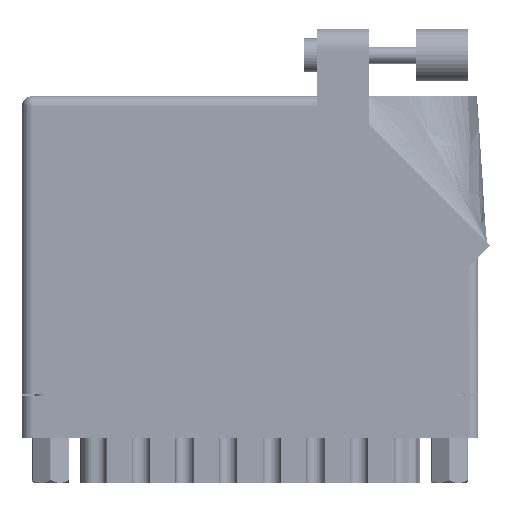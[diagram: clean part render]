
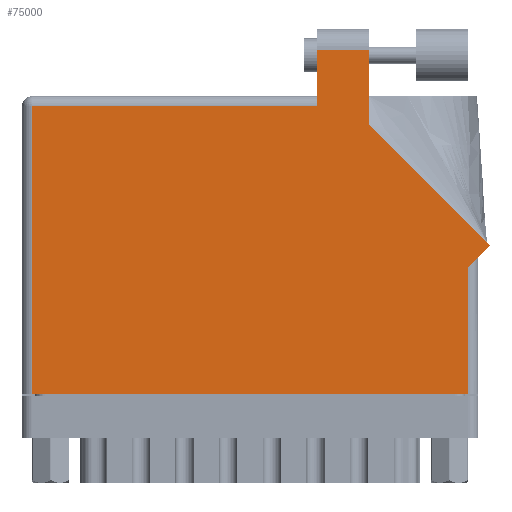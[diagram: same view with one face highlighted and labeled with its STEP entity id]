
A CAD part, front view. The second image highlights one B-rep face of the part: STEP entity #75000.
In plain terms, the highlighted face is planar.
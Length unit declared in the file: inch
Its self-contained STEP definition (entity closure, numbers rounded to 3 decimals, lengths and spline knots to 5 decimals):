
#145 = VERTEX_POINT ( 'NONE', #25677 ) ;
#604 = LINE ( 'NONE', #80345, #53760 ) ;
#2448 = ORIENTED_EDGE ( 'NONE', *, *, #78573, .T. ) ;
#3013 = DIRECTION ( 'NONE',  ( -1., 0., 0. ) ) ;
#3029 = VERTEX_POINT ( 'NONE', #69139 ) ;
#4702 = VECTOR ( 'NONE', #45036, 39.37008 ) ;
#5877 = VECTOR ( 'NONE', #77091, 39.37008 ) ;
#7147 = DIRECTION ( 'NONE',  ( 1., 0., 0. ) ) ;
#7571 = EDGE_CURVE ( 'NONE', #74211, #3029, #604, .T. ) ;
#8054 = EDGE_CURVE ( 'NONE', #48027, #145, #8754, .T. ) ;
#8754 = LINE ( 'NONE', #68455, #78065 ) ;
#9416 = CARTESIAN_POINT ( 'NONE',  ( 2.656, 0.753, 0. ) ) ;
#10268 = DIRECTION ( 'NONE',  ( 0., 1., 0. ) ) ;
#10323 = EDGE_CURVE ( 'NONE', #145, #74211, #11281, .T. ) ;
#11281 = LINE ( 'NONE', #75787, #5877 ) ;
#12767 = ORIENTED_EDGE ( 'NONE', *, *, #10323, .T. ) ;
#13566 = PLANE ( 'NONE',  #34576 ) ;
#14082 = CARTESIAN_POINT ( 'NONE',  ( 1.758, 2.05, 0. ) ) ;
#14623 = VECTOR ( 'NONE', #31779, 39.37008 ) ;
#18066 = VECTOR ( 'NONE', #33935, 39.37008 ) ;
#21176 = CARTESIAN_POINT ( 'NONE',  ( 0.062, 0., 0. ) ) ;
#21642 = VERTEX_POINT ( 'NONE', #9416 ) ;
#22251 = EDGE_CURVE ( 'NONE', #45679, #64475, #58549, .T. ) ;
#24321 = CARTESIAN_POINT ( 'NONE',  ( 2.78871, 0.88571, 0. ) ) ;
#25677 = CARTESIAN_POINT ( 'NONE',  ( 0.062, 1.713, 0. ) ) ;
#25924 = ORIENTED_EDGE ( 'NONE', *, *, #64978, .T. ) ;
#27938 = VECTOR ( 'NONE', #40461, 39.37008 ) ;
#29356 = ORIENTED_EDGE ( 'NONE', *, *, #58772, .T. ) ;
#31779 = DIRECTION ( 'NONE',  ( 0., -1., 0. ) ) ;
#33322 = CARTESIAN_POINT ( 'NONE',  ( 2.065, 1.60942, 0. ) ) ;
#33623 = DIRECTION ( 'NONE',  ( -1., 0., 0. ) ) ;
#33935 = DIRECTION ( 'NONE',  ( 0., 1., 0. ) ) ;
#34576 = AXIS2_PLACEMENT_3D ( 'NONE', #40179, #66745, #41039 ) ;
#40179 = CARTESIAN_POINT ( 'NONE',  ( 0., 1.775, 0. ) ) ;
#40461 = DIRECTION ( 'NONE',  ( 0.707, 0.707, 0. ) ) ;
#40762 = ORIENTED_EDGE ( 'NONE', *, *, #22251, .T. ) ;
#41039 = DIRECTION ( 'NONE',  ( -1., 0., 0. ) ) ;
#41055 = CARTESIAN_POINT ( 'NONE',  ( 1.758, 2.05, 0. ) ) ;
#42190 = LINE ( 'NONE', #80963, #27938 ) ;
#45012 = ORIENTED_EDGE ( 'NONE', *, *, #82156, .T. ) ;
#45036 = DIRECTION ( 'NONE',  ( -0.707, 0.707, 0. ) ) ;
#45679 = VERTEX_POINT ( 'NONE', #24321 ) ;
#46303 = CARTESIAN_POINT ( 'NONE',  ( 2.78871, 0.88571, 0. ) ) ;
#46749 = ORIENTED_EDGE ( 'NONE', *, *, #49122, .T. ) ;
#47156 = LINE ( 'NONE', #41055, #52067 ) ;
#48027 = VERTEX_POINT ( 'NONE', #61003 ) ;
#48297 = LINE ( 'NONE', #61377, #18066 ) ;
#49122 = EDGE_CURVE ( 'NONE', #67069, #48027, #63629, .T. ) ;
#52067 = VECTOR ( 'NONE', #3013, 39.37008 ) ;
#52515 = ORIENTED_EDGE ( 'NONE', *, *, #7571, .T. ) ;
#53760 = VECTOR ( 'NONE', #7147, 39.37008 ) ;
#54458 = VERTEX_POINT ( 'NONE', #57345 ) ;
#57345 = CARTESIAN_POINT ( 'NONE',  ( 2.065, 2.05, 0. ) ) ;
#58549 = LINE ( 'NONE', #46303, #4702 ) ;
#58772 = EDGE_CURVE ( 'NONE', #54458, #67069, #47156, .T. ) ;
#61003 = CARTESIAN_POINT ( 'NONE',  ( 1.758, 1.713, 0. ) ) ;
#61377 = CARTESIAN_POINT ( 'NONE',  ( 2.656, 0.815, 0. ) ) ;
#63629 = LINE ( 'NONE', #83663, #14623 ) ;
#64475 = VERTEX_POINT ( 'NONE', #33322 ) ;
#64978 = EDGE_CURVE ( 'NONE', #21642, #45679, #42190, .T. ) ;
#65840 = VECTOR ( 'NONE', #10268, 39.37008 ) ;
#66745 = DIRECTION ( 'NONE',  ( 0., 0., -1. ) ) ;
#67069 = VERTEX_POINT ( 'NONE', #14082 ) ;
#68455 = CARTESIAN_POINT ( 'NONE',  ( 0., 1.713, 0. ) ) ;
#69139 = CARTESIAN_POINT ( 'NONE',  ( 2.656, 0., 0. ) ) ;
#70384 = LINE ( 'NONE', #83901, #65840 ) ;
#74211 = VERTEX_POINT ( 'NONE', #21176 ) ;
#75000 = ADVANCED_FACE ( 'NONE', ( #79824 ), #13566, .F. ) ;
#75787 = CARTESIAN_POINT ( 'NONE',  ( 0.062, 0., 0. ) ) ;
#77091 = DIRECTION ( 'NONE',  ( 0., -1., 0. ) ) ;
#78065 = VECTOR ( 'NONE', #33623, 39.37008 ) ;
#78573 = EDGE_CURVE ( 'NONE', #3029, #21642, #48297, .T. ) ;
#79350 = EDGE_LOOP ( 'NONE', ( #45012, #29356, #46749, #80478, #12767, #52515, #2448, #25924, #40762 ) ) ;
#79824 = FACE_OUTER_BOUND ( 'NONE', #79350, .T. ) ;
#80345 = CARTESIAN_POINT ( 'NONE',  ( 0., 0., 0. ) ) ;
#80478 = ORIENTED_EDGE ( 'NONE', *, *, #8054, .T. ) ;
#80963 = CARTESIAN_POINT ( 'NONE',  ( 2.718, 0.815, 0. ) ) ;
#82156 = EDGE_CURVE ( 'NONE', #64475, #54458, #70384, .T. ) ;
#83663 = CARTESIAN_POINT ( 'NONE',  ( 1.758, 1.775, 0. ) ) ;
#83901 = CARTESIAN_POINT ( 'NONE',  ( 2.065, 1.60942, 0. ) ) ;
